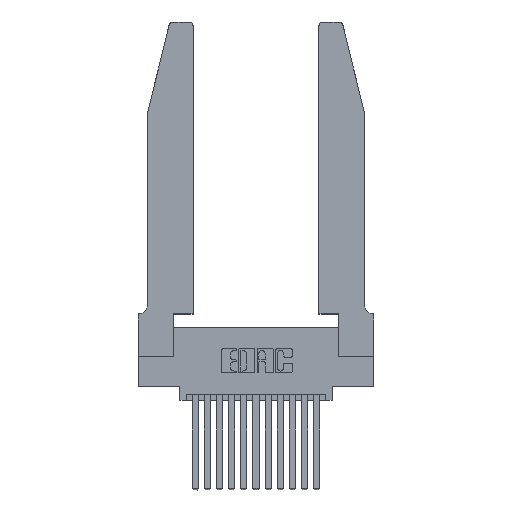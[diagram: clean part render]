
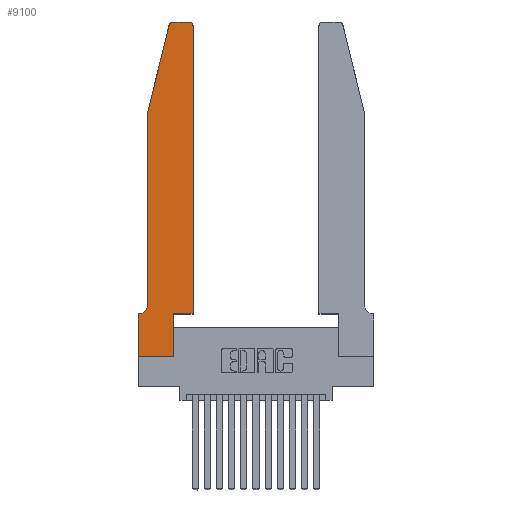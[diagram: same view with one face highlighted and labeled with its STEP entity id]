
A CAD part, top view. The second image highlights one B-rep face of the part: STEP entity #9100.
In plain terms, the highlighted planar face has unit normal (0, 0, 1).
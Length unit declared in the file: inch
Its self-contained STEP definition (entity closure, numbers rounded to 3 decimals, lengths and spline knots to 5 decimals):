
#180 = DIRECTION ( 'NONE',  ( -0.239, -0.971, 0. ) ) ;
#267 = VERTEX_POINT ( 'NONE', #878 ) ;
#292 = VECTOR ( 'NONE', #5067, 39.37008 ) ;
#710 = CARTESIAN_POINT ( 'NONE',  ( 0.2605, 2.75, 0.37 ) ) ;
#876 = CARTESIAN_POINT ( 'NONE',  ( 0.2865, 0.35, 0.37 ) ) ;
#878 = CARTESIAN_POINT ( 'NONE',  ( 0.0755, 2., 0.37 ) ) ;
#1173 = LINE ( 'NONE', #16078, #1597 ) ;
#1198 = AXIS2_PLACEMENT_3D ( 'NONE', #7180, #4288, #7051 ) ;
#1402 = EDGE_CURVE ( 'NONE', #5339, #8207, #16211, .T. ) ;
#1557 = LINE ( 'NONE', #2019, #10602 ) ;
#1597 = VECTOR ( 'NONE', #7795, 39.37008 ) ;
#1922 = VECTOR ( 'NONE', #180, 39.37008 ) ;
#2019 = CARTESIAN_POINT ( 'NONE',  ( 0., 0., 0.37 ) ) ;
#2020 = EDGE_CURVE ( 'NONE', #14006, #10445, #1557, .T. ) ;
#2183 = EDGE_CURVE ( 'NONE', #15172, #16624, #3867, .T. ) ;
#2850 = ORIENTED_EDGE ( 'NONE', *, *, #9529, .T. ) ;
#2998 = LINE ( 'NONE', #16386, #13789 ) ;
#3051 = CARTESIAN_POINT ( 'NONE',  ( 0.4205, 2.75, 0.37 ) ) ;
#3415 = DIRECTION ( 'NONE',  ( 1., 0., 0. ) ) ;
#3587 = ORIENTED_EDGE ( 'NONE', *, *, #1402, .T. ) ;
#3636 = EDGE_CURVE ( 'NONE', #5559, #14006, #1173, .T. ) ;
#3705 = CARTESIAN_POINT ( 'NONE',  ( 0.2865, 0., 0.37 ) ) ;
#3867 = LINE ( 'NONE', #6345, #292 ) ;
#4039 = AXIS2_PLACEMENT_3D ( 'NONE', #5224, #14645, #5158 ) ;
#4207 = ORIENTED_EDGE ( 'NONE', *, *, #9380, .T. ) ;
#4220 = VECTOR ( 'NONE', #16970, 39.37008 ) ;
#4288 = DIRECTION ( 'NONE',  ( 0., 0., -1. ) ) ;
#4318 = ORIENTED_EDGE ( 'NONE', *, *, #7100, .T. ) ;
#4635 = VECTOR ( 'NONE', #7237, 39.37008 ) ;
#5067 = DIRECTION ( 'NONE',  ( 1., 0., 0. ) ) ;
#5158 = DIRECTION ( 'NONE',  ( 1., 0., 0. ) ) ;
#5224 = CARTESIAN_POINT ( 'NONE',  ( 0.4205, 2.72, 0.37 ) ) ;
#5339 = VERTEX_POINT ( 'NONE', #13071 ) ;
#5395 = EDGE_CURVE ( 'NONE', #10445, #15172, #2998, .T. ) ;
#5559 = VERTEX_POINT ( 'NONE', #12499 ) ;
#5722 = CARTESIAN_POINT ( 'NONE',  ( 0., 0., 0.37 ) ) ;
#5881 = CARTESIAN_POINT ( 'NONE',  ( 0.0755, 0.35, 0.37 ) ) ;
#6244 = DIRECTION ( 'NONE',  ( 1., 0., 0. ) ) ;
#6337 = EDGE_CURVE ( 'NONE', #16624, #11363, #11415, .T. ) ;
#6345 = CARTESIAN_POINT ( 'NONE',  ( 0.4505, 0.35, 0.37 ) ) ;
#6751 = CARTESIAN_POINT ( 'NONE',  ( 0.0055, 0.35, 0.37 ) ) ;
#6854 = EDGE_CURVE ( 'NONE', #8207, #267, #10114, .T. ) ;
#6961 = DIRECTION ( 'NONE',  ( 1., 0., 0. ) ) ;
#7031 = EDGE_CURVE ( 'NONE', #8802, #10642, #15879, .T. ) ;
#7051 = DIRECTION ( 'NONE',  ( -1., 0., 0. ) ) ;
#7100 = EDGE_CURVE ( 'NONE', #10642, #5559, #12673, .T. ) ;
#7180 = CARTESIAN_POINT ( 'NONE',  ( 0.0055, 0.42, 0.37 ) ) ;
#7237 = DIRECTION ( 'NONE',  ( -1., 0., 0. ) ) ;
#7293 = ORIENTED_EDGE ( 'NONE', *, *, #5395, .T. ) ;
#7768 = CARTESIAN_POINT ( 'NONE',  ( 0.4505, 0.35, 0.37 ) ) ;
#7795 = DIRECTION ( 'NONE',  ( 0., -1., 0. ) ) ;
#7885 = AXIS2_PLACEMENT_3D ( 'NONE', #11620, #14213, #6244 ) ;
#7908 = ORIENTED_EDGE ( 'NONE', *, *, #2020, .T. ) ;
#8008 = CARTESIAN_POINT ( 'NONE',  ( 0.0755, 2., 0.37 ) ) ;
#8207 = VERTEX_POINT ( 'NONE', #14824 ) ;
#8309 = FACE_OUTER_BOUND ( 'NONE', #8596, .T. ) ;
#8596 = EDGE_LOOP ( 'NONE', ( #4207, #3587, #11546, #11400, #11544, #4318, #9139, #7908, #7293, #11018, #16506, #2850 ) ) ;
#8802 = VERTEX_POINT ( 'NONE', #9835 ) ;
#9100 = ADVANCED_FACE ( 'NONE', ( #8309 ), #9567, .T. ) ;
#9139 = ORIENTED_EDGE ( 'NONE', *, *, #3636, .T. ) ;
#9256 = DIRECTION ( 'NONE',  ( 0., -1., 0. ) ) ;
#9380 = EDGE_CURVE ( 'NONE', #10759, #5339, #15553, .T. ) ;
#9529 = EDGE_CURVE ( 'NONE', #11363, #10759, #16832, .T. ) ;
#9567 = PLANE ( 'NONE',  #13122 ) ;
#9835 = CARTESIAN_POINT ( 'NONE',  ( 0.0755, 0.42, 0.37 ) ) ;
#10114 = LINE ( 'NONE', #14917, #1922 ) ;
#10445 = VERTEX_POINT ( 'NONE', #3705 ) ;
#10602 = VECTOR ( 'NONE', #3415, 39.37008 ) ;
#10642 = VERTEX_POINT ( 'NONE', #6751 ) ;
#10759 = VERTEX_POINT ( 'NONE', #3051 ) ;
#11018 = ORIENTED_EDGE ( 'NONE', *, *, #2183, .T. ) ;
#11363 = VERTEX_POINT ( 'NONE', #13772 ) ;
#11400 = ORIENTED_EDGE ( 'NONE', *, *, #14738, .T. ) ;
#11415 = LINE ( 'NONE', #11635, #4220 ) ;
#11437 = DIRECTION ( 'NONE',  ( -1., 0., 0. ) ) ;
#11544 = ORIENTED_EDGE ( 'NONE', *, *, #7031, .T. ) ;
#11546 = ORIENTED_EDGE ( 'NONE', *, *, #6854, .T. ) ;
#11620 = CARTESIAN_POINT ( 'NONE',  ( 0.284, 2.72, 0.37 ) ) ;
#11635 = CARTESIAN_POINT ( 'NONE',  ( 0.4505, 0.35, 0.37 ) ) ;
#11891 = VECTOR ( 'NONE', #11437, 39.37008 ) ;
#12499 = CARTESIAN_POINT ( 'NONE',  ( 0., 0.35, 0.37 ) ) ;
#12673 = LINE ( 'NONE', #5881, #4635 ) ;
#12838 = LINE ( 'NONE', #8008, #13059 ) ;
#13059 = VECTOR ( 'NONE', #9256, 39.37008 ) ;
#13071 = CARTESIAN_POINT ( 'NONE',  ( 0.284, 2.75, 0.37 ) ) ;
#13122 = AXIS2_PLACEMENT_3D ( 'NONE', #16541, #16593, #6961 ) ;
#13577 = DIRECTION ( 'NONE',  ( 0., 1., 0. ) ) ;
#13772 = CARTESIAN_POINT ( 'NONE',  ( 0.4505, 2.72, 0.37 ) ) ;
#13789 = VECTOR ( 'NONE', #13577, 39.37008 ) ;
#14006 = VERTEX_POINT ( 'NONE', #5722 ) ;
#14213 = DIRECTION ( 'NONE',  ( 0., 0., 1. ) ) ;
#14645 = DIRECTION ( 'NONE',  ( 0., 0., 1. ) ) ;
#14738 = EDGE_CURVE ( 'NONE', #267, #8802, #12838, .T. ) ;
#14824 = CARTESIAN_POINT ( 'NONE',  ( 0.25487, 2.72718, 0.37 ) ) ;
#14917 = CARTESIAN_POINT ( 'NONE',  ( 0.0755, 2., 0.37 ) ) ;
#15172 = VERTEX_POINT ( 'NONE', #876 ) ;
#15553 = LINE ( 'NONE', #710, #11891 ) ;
#15879 = CIRCLE ( 'NONE', #1198, 0.07 ) ;
#16078 = CARTESIAN_POINT ( 'NONE',  ( 0., 0., 0.37 ) ) ;
#16211 = CIRCLE ( 'NONE', #7885, 0.03 ) ;
#16386 = CARTESIAN_POINT ( 'NONE',  ( 0.2865, 0.35, 0.37 ) ) ;
#16506 = ORIENTED_EDGE ( 'NONE', *, *, #6337, .T. ) ;
#16541 = CARTESIAN_POINT ( 'NONE',  ( 0., 0.35, 0.37 ) ) ;
#16593 = DIRECTION ( 'NONE',  ( 0., 0., 1. ) ) ;
#16624 = VERTEX_POINT ( 'NONE', #7768 ) ;
#16832 = CIRCLE ( 'NONE', #4039, 0.03 ) ;
#16970 = DIRECTION ( 'NONE',  ( 0., 1., 0. ) ) ;
